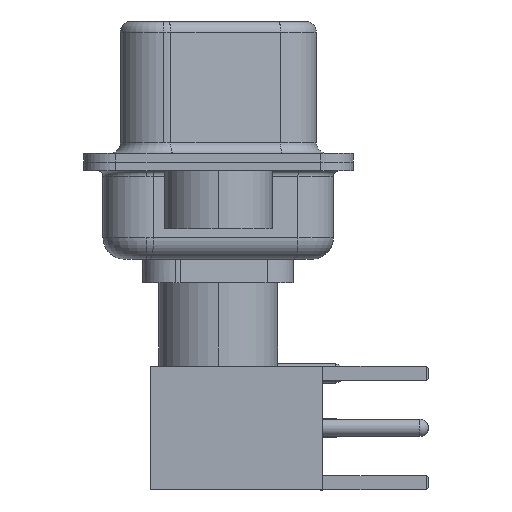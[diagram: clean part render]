
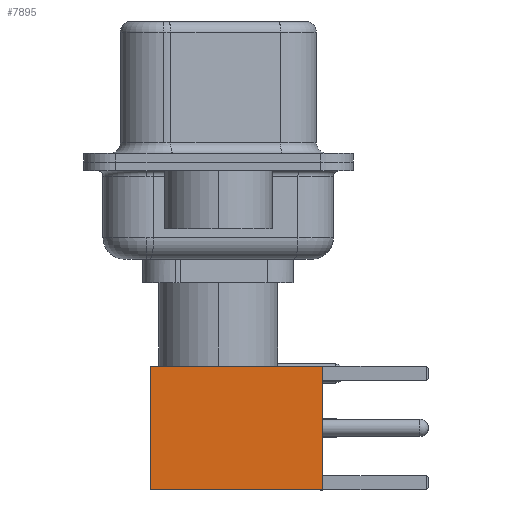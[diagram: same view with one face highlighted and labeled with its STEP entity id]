
A CAD part, left-side view. The second image highlights one B-rep face of the part: STEP entity #7895.
In plain terms, the highlighted face is planar.
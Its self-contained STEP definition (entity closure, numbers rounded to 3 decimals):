
#837 = ORIENTED_EDGE ( 'NONE', *, *, #4139, .T. ) ;
#1084 = VERTEX_POINT ( 'NONE', #24104 ) ;
#1493 = LINE ( 'NONE', #4092, #20923 ) ;
#2549 = LINE ( 'NONE', #16988, #4017 ) ;
#3466 = VERTEX_POINT ( 'NONE', #11114 ) ;
#3655 = DIRECTION ( 'NONE',  ( 0., 1., 0. ) ) ;
#3800 = FACE_OUTER_BOUND ( 'NONE', #27293, .T. ) ;
#3871 = LINE ( 'NONE', #29565, #24828 ) ;
#3980 = ORIENTED_EDGE ( 'NONE', *, *, #5621, .T. ) ;
#4017 = VECTOR ( 'NONE', #11987, 1000. ) ;
#4092 = CARTESIAN_POINT ( 'NONE',  ( 0., 2.875, 8. ) ) ;
#4139 = EDGE_CURVE ( 'NONE', #3466, #24324, #2549, .T. ) ;
#4690 = CARTESIAN_POINT ( 'NONE',  ( 2.875, 2.875, 0. ) ) ;
#5621 = EDGE_CURVE ( 'NONE', #24324, #1084, #3871, .T. ) ;
#6812 = CARTESIAN_POINT ( 'NONE',  ( -2.875, 2.875, 0. ) ) ;
#7895 = ADVANCED_FACE ( 'NONE', ( #3800 ), #17949, .T. ) ;
#8789 = DIRECTION ( 'NONE',  ( 0., 0., -1. ) ) ;
#9901 = CARTESIAN_POINT ( 'NONE',  ( -2.875, 2.875, 8. ) ) ;
#10113 = VECTOR ( 'NONE', #8789, 1000. ) ;
#10499 = DIRECTION ( 'NONE',  ( -1., 0., 0. ) ) ;
#11114 = CARTESIAN_POINT ( 'NONE',  ( 2.875, 2.875, 8. ) ) ;
#11987 = DIRECTION ( 'NONE',  ( 0., 0., -1. ) ) ;
#12602 = EDGE_CURVE ( 'NONE', #20927, #1084, #15925, .T. ) ;
#13242 = DIRECTION ( 'NONE',  ( 0., 0., 1. ) ) ;
#15925 = LINE ( 'NONE', #6812, #10113 ) ;
#16907 = EDGE_CURVE ( 'NONE', #3466, #20927, #1493, .T. ) ;
#16988 = CARTESIAN_POINT ( 'NONE',  ( 2.875, 2.875, 0. ) ) ;
#17143 = ORIENTED_EDGE ( 'NONE', *, *, #12602, .F. ) ;
#17949 = PLANE ( 'NONE',  #27394 ) ;
#18014 = DIRECTION ( 'NONE',  ( -1., 0., 0. ) ) ;
#20923 = VECTOR ( 'NONE', #10499, 1000. ) ;
#20927 = VERTEX_POINT ( 'NONE', #9901 ) ;
#24104 = CARTESIAN_POINT ( 'NONE',  ( -2.875, 2.875, 0. ) ) ;
#24324 = VERTEX_POINT ( 'NONE', #4690 ) ;
#24828 = VECTOR ( 'NONE', #18014, 1000. ) ;
#27231 = CARTESIAN_POINT ( 'NONE',  ( 2.875, 2.875, 0. ) ) ;
#27293 = EDGE_LOOP ( 'NONE', ( #837, #3980, #17143, #29417 ) ) ;
#27394 = AXIS2_PLACEMENT_3D ( 'NONE', #27231, #3655, #13242 ) ;
#29417 = ORIENTED_EDGE ( 'NONE', *, *, #16907, .F. ) ;
#29565 = CARTESIAN_POINT ( 'NONE',  ( 0., 2.875, 0. ) ) ;
